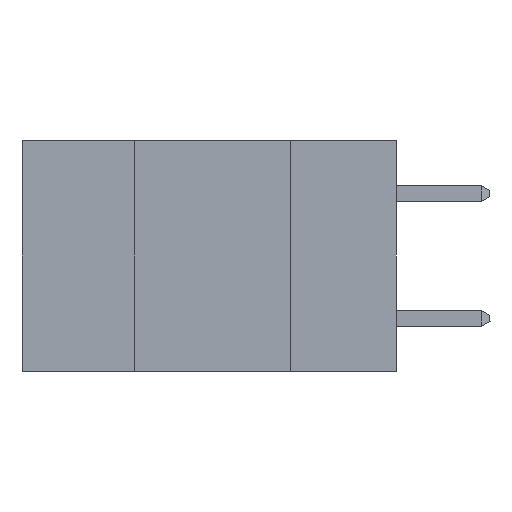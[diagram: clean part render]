
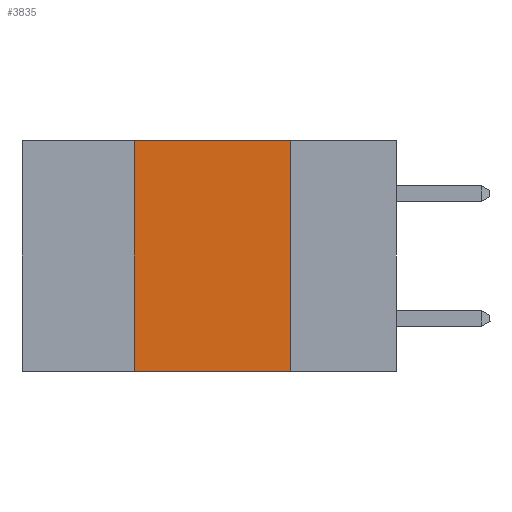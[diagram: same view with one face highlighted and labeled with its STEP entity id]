
A CAD part, left-side view. The second image highlights one B-rep face of the part: STEP entity #3835.
In plain terms, the highlighted planar face has unit normal (-1, 0, 0).
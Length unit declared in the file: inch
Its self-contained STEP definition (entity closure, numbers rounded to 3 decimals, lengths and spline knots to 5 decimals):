
#148 = FACE_OUTER_BOUND ( 'NONE', #10704, .T. ) ;
#1044 = CARTESIAN_POINT ( 'NONE',  ( 0., 0.42, -0.37 ) ) ;
#1379 = EDGE_CURVE ( 'NONE', #22997, #4075, #21613, .T. ) ;
#1541 = VECTOR ( 'NONE', #10260, 39.37008 ) ;
#1936 = CARTESIAN_POINT ( 'NONE',  ( 0., 0.17, -0.37 ) ) ;
#2960 = CARTESIAN_POINT ( 'NONE',  ( 0., 0.42, -0.37 ) ) ;
#3069 = DIRECTION ( 'NONE',  ( 0., 0., -1. ) ) ;
#3074 = DIRECTION ( 'NONE',  ( 1., 0., 0. ) ) ;
#3179 = CARTESIAN_POINT ( 'NONE',  ( 0., 0.6, 0. ) ) ;
#3290 = PLANE ( 'NONE',  #12694 ) ;
#3835 = ADVANCED_FACE ( 'NONE', ( #148 ), #3290, .F. ) ;
#4075 = VERTEX_POINT ( 'NONE', #1936 ) ;
#4273 = CARTESIAN_POINT ( 'NONE',  ( 0., 0.6, -0.37 ) ) ;
#4901 = VECTOR ( 'NONE', #14230, 39.37008 ) ;
#6010 = EDGE_CURVE ( 'NONE', #16762, #19398, #7177, .T. ) ;
#6491 = CARTESIAN_POINT ( 'NONE',  ( 0., 0.6, 0. ) ) ;
#6926 = LINE ( 'NONE', #19002, #22283 ) ;
#7177 = LINE ( 'NONE', #6491, #1541 ) ;
#7845 = DIRECTION ( 'NONE',  ( 0., 0., -1. ) ) ;
#9850 = EDGE_CURVE ( 'NONE', #22997, #16762, #10578, .T. ) ;
#10260 = DIRECTION ( 'NONE',  ( 0., -1., 0. ) ) ;
#10578 = LINE ( 'NONE', #1044, #4901 ) ;
#10704 = EDGE_LOOP ( 'NONE', ( #11680, #13685, #15068, #12246 ) ) ;
#11248 = CARTESIAN_POINT ( 'NONE',  ( 0., 0.17, 0. ) ) ;
#11680 = ORIENTED_EDGE ( 'NONE', *, *, #16119, .F. ) ;
#11883 = VECTOR ( 'NONE', #16582, 39.37008 ) ;
#12246 = ORIENTED_EDGE ( 'NONE', *, *, #1379, .T. ) ;
#12694 = AXIS2_PLACEMENT_3D ( 'NONE', #3179, #3074, #3069 ) ;
#13685 = ORIENTED_EDGE ( 'NONE', *, *, #6010, .F. ) ;
#13841 = CARTESIAN_POINT ( 'NONE',  ( 0., 0.42, 0. ) ) ;
#14230 = DIRECTION ( 'NONE',  ( 0., 0., 1. ) ) ;
#15068 = ORIENTED_EDGE ( 'NONE', *, *, #9850, .F. ) ;
#16119 = EDGE_CURVE ( 'NONE', #19398, #4075, #6926, .T. ) ;
#16582 = DIRECTION ( 'NONE',  ( 0., -1., 0. ) ) ;
#16762 = VERTEX_POINT ( 'NONE', #13841 ) ;
#19002 = CARTESIAN_POINT ( 'NONE',  ( 0., 0.17, -0.37 ) ) ;
#19398 = VERTEX_POINT ( 'NONE', #11248 ) ;
#21613 = LINE ( 'NONE', #4273, #11883 ) ;
#22283 = VECTOR ( 'NONE', #7845, 39.37008 ) ;
#22997 = VERTEX_POINT ( 'NONE', #2960 ) ;
